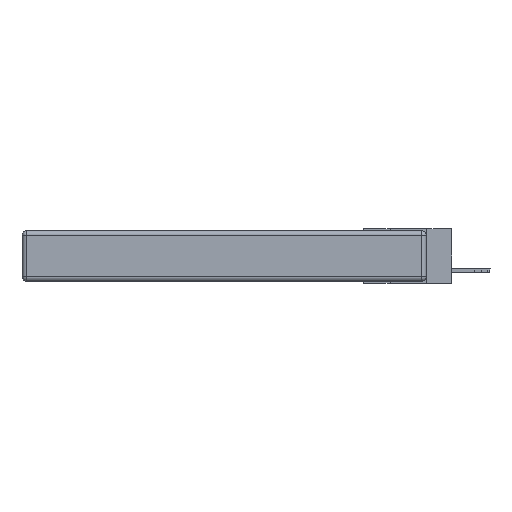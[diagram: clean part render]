
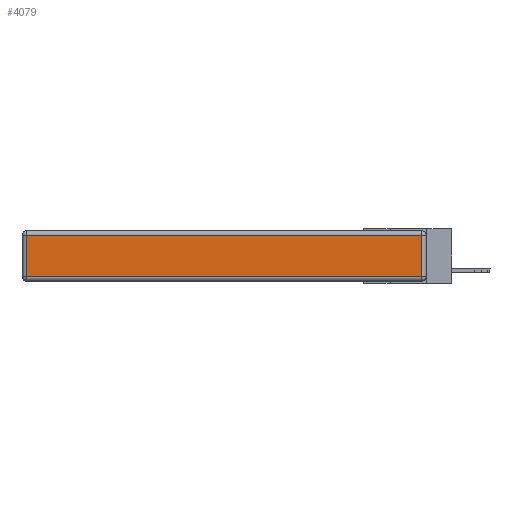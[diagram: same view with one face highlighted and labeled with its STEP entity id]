
A CAD part, left-side view. The second image highlights one B-rep face of the part: STEP entity #4079.
In plain terms, the highlighted planar face has unit normal (-1, 0, 0).
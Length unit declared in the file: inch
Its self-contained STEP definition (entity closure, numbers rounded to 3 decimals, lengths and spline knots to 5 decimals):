
#169 = DIRECTION ( 'NONE',  ( -1., 0., 0. ) ) ;
#176 = CARTESIAN_POINT ( 'NONE',  ( 0., 2.75, -0.03 ) ) ;
#712 = ORIENTED_EDGE ( 'NONE', *, *, #14719, .T. ) ;
#780 = CARTESIAN_POINT ( 'NONE',  ( 0., 0., -0.313 ) ) ;
#789 = AXIS2_PLACEMENT_3D ( 'NONE', #1435, #169, #7011 ) ;
#900 = ORIENTED_EDGE ( 'NONE', *, *, #7727, .T. ) ;
#1435 = CARTESIAN_POINT ( 'NONE',  ( 0., 0., -0.343 ) ) ;
#1531 = VECTOR ( 'NONE', #9417, 39.37008 ) ;
#2318 = CARTESIAN_POINT ( 'NONE',  ( 0., 2.72, -0.313 ) ) ;
#2530 = VERTEX_POINT ( 'NONE', #12237 ) ;
#2789 = LINE ( 'NONE', #780, #12563 ) ;
#2864 = LINE ( 'NONE', #2985, #14128 ) ;
#2962 = LINE ( 'NONE', #14081, #1531 ) ;
#2985 = CARTESIAN_POINT ( 'NONE',  ( 0., 2.72, -0.343 ) ) ;
#3681 = PLANE ( 'NONE',  #789 ) ;
#3909 = EDGE_LOOP ( 'NONE', ( #900, #712, #14987, #11432 ) ) ;
#4079 = ADVANCED_FACE ( 'NONE', ( #14415 ), #3681, .T. ) ;
#4230 = DIRECTION ( 'NONE',  ( 0., -1., 0. ) ) ;
#4357 = VERTEX_POINT ( 'NONE', #7470 ) ;
#4484 = VERTEX_POINT ( 'NONE', #2318 ) ;
#6536 = EDGE_CURVE ( 'NONE', #4357, #6961, #7955, .T. ) ;
#6961 = VERTEX_POINT ( 'NONE', #13055 ) ;
#7011 = DIRECTION ( 'NONE',  ( 0., 0., 1. ) ) ;
#7164 = DIRECTION ( 'NONE',  ( 0., 1., 0. ) ) ;
#7470 = CARTESIAN_POINT ( 'NONE',  ( 0., 0.03, -0.03 ) ) ;
#7727 = EDGE_CURVE ( 'NONE', #4484, #2530, #2789, .T. ) ;
#7955 = LINE ( 'NONE', #176, #12290 ) ;
#9417 = DIRECTION ( 'NONE',  ( 0., 0., 1. ) ) ;
#10586 = EDGE_CURVE ( 'NONE', #6961, #4484, #2864, .T. ) ;
#11432 = ORIENTED_EDGE ( 'NONE', *, *, #10586, .T. ) ;
#12127 = DIRECTION ( 'NONE',  ( 0., 0., -1. ) ) ;
#12237 = CARTESIAN_POINT ( 'NONE',  ( 0., 0.03, -0.313 ) ) ;
#12290 = VECTOR ( 'NONE', #7164, 39.37008 ) ;
#12563 = VECTOR ( 'NONE', #4230, 39.37008 ) ;
#13055 = CARTESIAN_POINT ( 'NONE',  ( 0., 2.72, -0.03 ) ) ;
#14081 = CARTESIAN_POINT ( 'NONE',  ( 0., 0.03, -0.343 ) ) ;
#14128 = VECTOR ( 'NONE', #12127, 39.37008 ) ;
#14415 = FACE_OUTER_BOUND ( 'NONE', #3909, .T. ) ;
#14719 = EDGE_CURVE ( 'NONE', #2530, #4357, #2962, .T. ) ;
#14987 = ORIENTED_EDGE ( 'NONE', *, *, #6536, .T. ) ;
